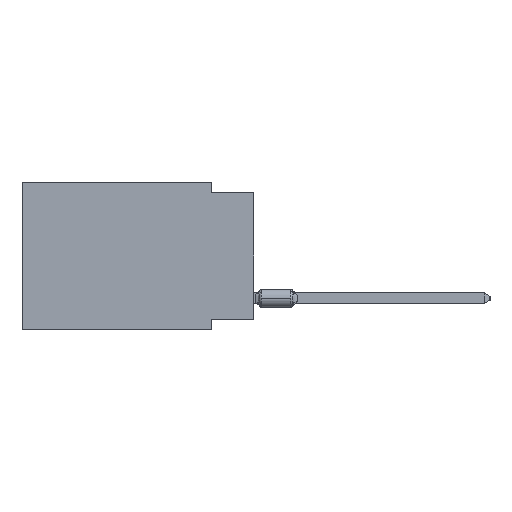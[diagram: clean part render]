
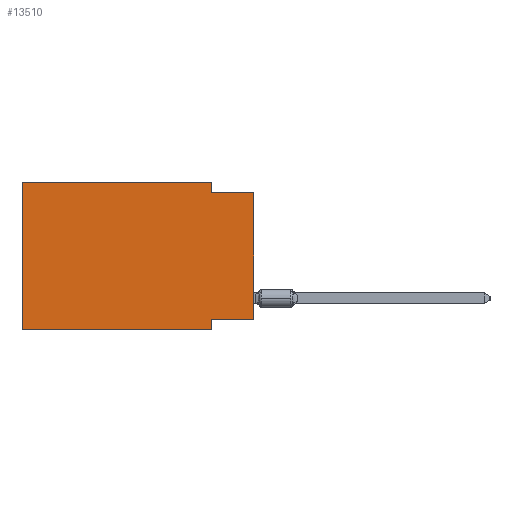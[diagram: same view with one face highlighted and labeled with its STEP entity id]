
A CAD part, left-side view. The second image highlights one B-rep face of the part: STEP entity #13510.
In plain terms, the highlighted planar face has unit normal (-1, 0, 0).
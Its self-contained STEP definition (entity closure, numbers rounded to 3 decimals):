
#158 = CARTESIAN_POINT ( 'NONE',  ( 0., 0., -8.255 ) ) ;
#347 = VECTOR ( 'NONE', #37968, 1000. ) ;
#3245 = CARTESIAN_POINT ( 'NONE',  ( 0., 2.54, 0. ) ) ;
#5438 = VERTEX_POINT ( 'NONE', #89598 ) ;
#6398 = ORIENTED_EDGE ( 'NONE', *, *, #33922, .F. ) ;
#7466 = CARTESIAN_POINT ( 'NONE',  ( 0., 13.97, 0. ) ) ;
#8366 = VERTEX_POINT ( 'NONE', #39747 ) ;
#9270 = LINE ( 'NONE', #87007, #32029 ) ;
#9455 = VECTOR ( 'NONE', #86920, 1000. ) ;
#13510 = ADVANCED_FACE ( 'NONE', ( #27675 ), #96192, .F. ) ;
#14862 = VERTEX_POINT ( 'NONE', #37390 ) ;
#15525 = EDGE_LOOP ( 'NONE', ( #94616, #49594, #6398, #26469, #79068, #39076, #99250, #57050 ) ) ;
#15532 = VERTEX_POINT ( 'NONE', #40152 ) ;
#18983 = DIRECTION ( 'NONE',  ( 1., 0., 0. ) ) ;
#19990 = DIRECTION ( 'NONE',  ( 0., 0., -1. ) ) ;
#22194 = VERTEX_POINT ( 'NONE', #62991 ) ;
#26469 = ORIENTED_EDGE ( 'NONE', *, *, #88886, .F. ) ;
#27104 = CARTESIAN_POINT ( 'NONE',  ( 0., 2.54, -8.89 ) ) ;
#27675 = FACE_OUTER_BOUND ( 'NONE', #15525, .T. ) ;
#30003 = LINE ( 'NONE', #7466, #40935 ) ;
#32029 = VECTOR ( 'NONE', #32336, 1000. ) ;
#32336 = DIRECTION ( 'NONE',  ( 0., -1., 0. ) ) ;
#33922 = EDGE_CURVE ( 'NONE', #5438, #15532, #88154, .T. ) ;
#34374 = CARTESIAN_POINT ( 'NONE',  ( 0., 13.97, 0. ) ) ;
#36585 = CARTESIAN_POINT ( 'NONE',  ( 0., 0., -0.635 ) ) ;
#37390 = CARTESIAN_POINT ( 'NONE',  ( 0., 2.54, -8.89 ) ) ;
#37968 = DIRECTION ( 'NONE',  ( 0., 0., 1. ) ) ;
#38697 = DIRECTION ( 'NONE',  ( 0., -1., 0. ) ) ;
#39076 = ORIENTED_EDGE ( 'NONE', *, *, #85897, .T. ) ;
#39747 = CARTESIAN_POINT ( 'NONE',  ( 0., 13.97, 0. ) ) ;
#40152 = CARTESIAN_POINT ( 'NONE',  ( 0., 2.54, -0.635 ) ) ;
#40935 = VECTOR ( 'NONE', #38697, 1000. ) ;
#43103 = EDGE_CURVE ( 'NONE', #22194, #14862, #73640, .T. ) ;
#46867 = CARTESIAN_POINT ( 'NONE',  ( 0., 13.97, 0. ) ) ;
#47922 = EDGE_CURVE ( 'NONE', #100871, #8366, #65594, .T. ) ;
#48263 = EDGE_CURVE ( 'NONE', #60664, #98803, #76797, .T. ) ;
#49415 = VECTOR ( 'NONE', #77881, 1000. ) ;
#49594 = ORIENTED_EDGE ( 'NONE', *, *, #82446, .F. ) ;
#51674 = VECTOR ( 'NONE', #82299, 1000. ) ;
#57050 = ORIENTED_EDGE ( 'NONE', *, *, #69390, .F. ) ;
#60664 = VERTEX_POINT ( 'NONE', #92433 ) ;
#62991 = CARTESIAN_POINT ( 'NONE',  ( 0., 2.54, -8.255 ) ) ;
#64047 = LINE ( 'NONE', #158, #49415 ) ;
#65594 = LINE ( 'NONE', #46867, #73732 ) ;
#69390 = EDGE_CURVE ( 'NONE', #60664, #22194, #64047, .T. ) ;
#73640 = LINE ( 'NONE', #27104, #51674 ) ;
#73732 = VECTOR ( 'NONE', #86236, 1000. ) ;
#76797 = LINE ( 'NONE', #100794, #347 ) ;
#77881 = DIRECTION ( 'NONE',  ( 0., 1., 0. ) ) ;
#78741 = CARTESIAN_POINT ( 'NONE',  ( 0., 13.97, -8.89 ) ) ;
#79068 = ORIENTED_EDGE ( 'NONE', *, *, #47922, .F. ) ;
#80359 = CARTESIAN_POINT ( 'NONE',  ( 0., 13.97, -8.89 ) ) ;
#81217 = AXIS2_PLACEMENT_3D ( 'NONE', #34374, #18983, #19990 ) ;
#82299 = DIRECTION ( 'NONE',  ( 0., 0., -1. ) ) ;
#82446 = EDGE_CURVE ( 'NONE', #15532, #98803, #9270, .T. ) ;
#85897 = EDGE_CURVE ( 'NONE', #100871, #14862, #86415, .T. ) ;
#86236 = DIRECTION ( 'NONE',  ( 0., 0., 1. ) ) ;
#86415 = LINE ( 'NONE', #78741, #9455 ) ;
#86920 = DIRECTION ( 'NONE',  ( 0., -1., 0. ) ) ;
#87007 = CARTESIAN_POINT ( 'NONE',  ( 0., 0., -0.635 ) ) ;
#88154 = LINE ( 'NONE', #3245, #93015 ) ;
#88886 = EDGE_CURVE ( 'NONE', #8366, #5438, #30003, .T. ) ;
#89598 = CARTESIAN_POINT ( 'NONE',  ( 0., 2.54, 0. ) ) ;
#92433 = CARTESIAN_POINT ( 'NONE',  ( 0., 0., -8.255 ) ) ;
#93015 = VECTOR ( 'NONE', #95792, 1000. ) ;
#94616 = ORIENTED_EDGE ( 'NONE', *, *, #48263, .T. ) ;
#95792 = DIRECTION ( 'NONE',  ( 0., 0., -1. ) ) ;
#96192 = PLANE ( 'NONE',  #81217 ) ;
#98803 = VERTEX_POINT ( 'NONE', #36585 ) ;
#99250 = ORIENTED_EDGE ( 'NONE', *, *, #43103, .F. ) ;
#100794 = CARTESIAN_POINT ( 'NONE',  ( 0., 0., 0. ) ) ;
#100871 = VERTEX_POINT ( 'NONE', #80359 ) ;
